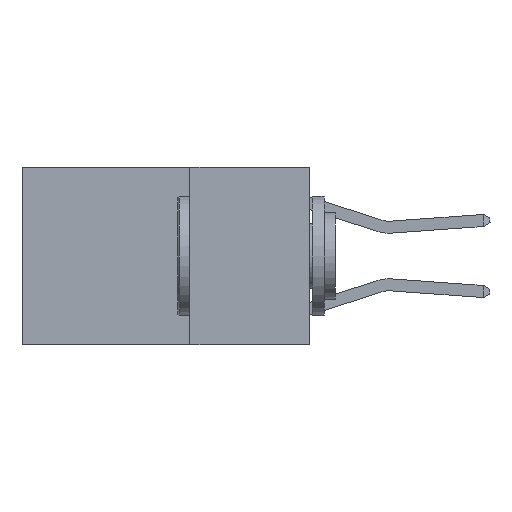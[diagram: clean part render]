
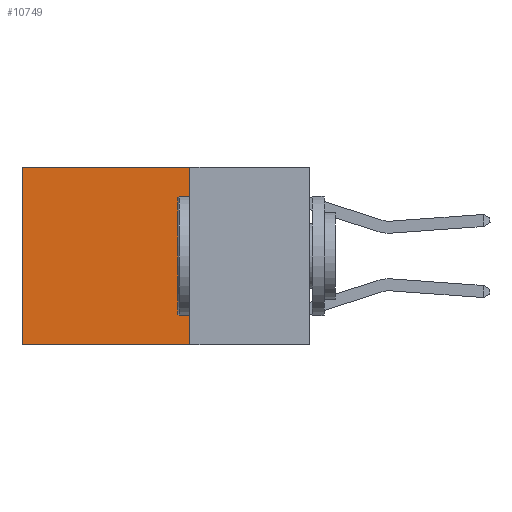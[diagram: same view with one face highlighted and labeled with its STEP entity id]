
A CAD part, left-side view. The second image highlights one B-rep face of the part: STEP entity #10749.
In plain terms, the highlighted planar face has unit normal (-1, 0, 0).
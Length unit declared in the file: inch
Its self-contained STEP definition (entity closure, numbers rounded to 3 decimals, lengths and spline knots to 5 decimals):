
#912 = VERTEX_POINT ( 'NONE', #4932 ) ;
#942 = VECTOR ( 'NONE', #13205, 39.37008 ) ;
#2980 = PLANE ( 'NONE',  #16605 ) ;
#3060 = VECTOR ( 'NONE', #10545, 39.37008 ) ;
#3127 = ORIENTED_EDGE ( 'NONE', *, *, #15748, .T. ) ;
#3134 = ORIENTED_EDGE ( 'NONE', *, *, #13276, .F. ) ;
#3395 = DIRECTION ( 'NONE',  ( 0., 0., -1. ) ) ;
#3493 = LINE ( 'NONE', #13174, #3060 ) ;
#3646 = CARTESIAN_POINT ( 'NONE',  ( 0.2625, 0.25, 0. ) ) ;
#3693 = CARTESIAN_POINT ( 'NONE',  ( 0.2625, 0.6, 0. ) ) ;
#4126 = LINE ( 'NONE', #3646, #942 ) ;
#4342 = DIRECTION ( 'NONE',  ( 0., 0., -1. ) ) ;
#4932 = CARTESIAN_POINT ( 'NONE',  ( 0.2625, 0.25, -0.37 ) ) ;
#5858 = FACE_OUTER_BOUND ( 'NONE', #16350, .T. ) ;
#6756 = ORIENTED_EDGE ( 'NONE', *, *, #12058, .T. ) ;
#8423 = VERTEX_POINT ( 'NONE', #3693 ) ;
#9854 = CARTESIAN_POINT ( 'NONE',  ( 0.2625, 0.6, -0.37 ) ) ;
#10545 = DIRECTION ( 'NONE',  ( 0., 1., 0. ) ) ;
#10749 = ADVANCED_FACE ( 'NONE', ( #5858 ), #2980, .F. ) ;
#11013 = VECTOR ( 'NONE', #12289, 39.37008 ) ;
#11390 = EDGE_CURVE ( 'NONE', #912, #12454, #3493, .T. ) ;
#11716 = VERTEX_POINT ( 'NONE', #14130 ) ;
#11809 = VECTOR ( 'NONE', #3395, 39.37008 ) ;
#12058 = EDGE_CURVE ( 'NONE', #11716, #8423, #4126, .T. ) ;
#12225 = LINE ( 'NONE', #16659, #11809 ) ;
#12289 = DIRECTION ( 'NONE',  ( 0., 0., -1. ) ) ;
#12454 = VERTEX_POINT ( 'NONE', #9854 ) ;
#12598 = DIRECTION ( 'NONE',  ( 1., 0., 0. ) ) ;
#13174 = CARTESIAN_POINT ( 'NONE',  ( 0.2625, 0.25, -0.37 ) ) ;
#13205 = DIRECTION ( 'NONE',  ( 0., 1., 0. ) ) ;
#13276 = EDGE_CURVE ( 'NONE', #11716, #912, #14442, .T. ) ;
#14130 = CARTESIAN_POINT ( 'NONE',  ( 0.2625, 0.25, 0. ) ) ;
#14442 = LINE ( 'NONE', #17255, #11013 ) ;
#15044 = CARTESIAN_POINT ( 'NONE',  ( 0.2625, 0.25, 0. ) ) ;
#15748 = EDGE_CURVE ( 'NONE', #8423, #12454, #12225, .T. ) ;
#16350 = EDGE_LOOP ( 'NONE', ( #3127, #17263, #3134, #6756 ) ) ;
#16605 = AXIS2_PLACEMENT_3D ( 'NONE', #15044, #12598, #4342 ) ;
#16659 = CARTESIAN_POINT ( 'NONE',  ( 0.2625, 0.6, 0. ) ) ;
#17255 = CARTESIAN_POINT ( 'NONE',  ( 0.2625, 0.25, 0. ) ) ;
#17263 = ORIENTED_EDGE ( 'NONE', *, *, #11390, .F. ) ;
